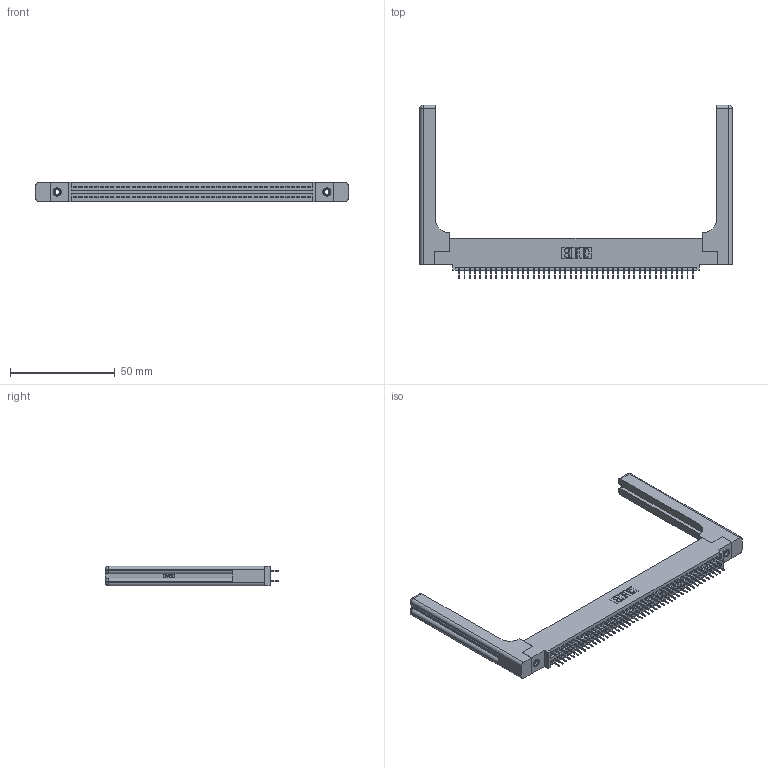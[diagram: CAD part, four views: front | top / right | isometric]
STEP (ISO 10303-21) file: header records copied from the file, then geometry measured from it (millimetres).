
FILE_DESCRIPTION (( 'STEP AP203' ), '1' );
FILE_NAME ('395-090-524-558.STEP', '2019-10-25T16:22:01', ( '' ), ( '' ), 'SwSTEP 2.0', 'SolidWorks 2016', '' );
FILE_SCHEMA (( 'CONFIG_CONTROL_DESIGN' ));
Length unit declared in the file: inch
Products named in the file (5): 345-220-058_345-220-058; 395-090-524-558; 345 Part_0.110 Offset - 0.156 Dia-TH; 345-292-001_345-293-124; 345-250-001_345-250-001-102
Assembly tree (95 placements, depth 2):
  395-090-524-558
    345 Part_0.110 Offset - 0.156 Dia-TH
    345-292-001_345-293-124  x90
    345-250-001_345-250-001-102  x2
    345-220-058_345-220-058  x2
Bounding box: 149.33 x 83.11 x 9.4 mm (x, y, z)
Volume: 22799.1 mm3; surface area: 26023.6 mm2
Topology: 95 solids, 95 shells, 5246 faces, 14789 edges, 9478 vertices
Faces by surface type: plane 3742, cylinder 1444, bspline 36, cone 12, sphere 8, torus 4
Entity records: 40292 total; most frequent: CARTESIAN_POINT 7745, ORIENTED_EDGE 6476, DIRECTION 5758, EDGE_CURVE 3238, VECTOR 2838, LINE 2838, VERTEX_POINT 2146, AXIS2_PLACEMENT_3D 1460
